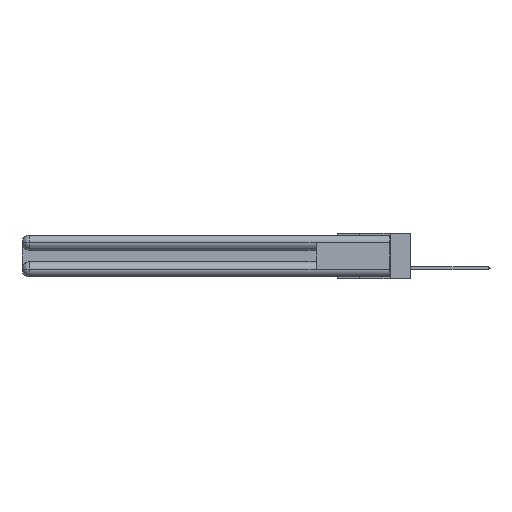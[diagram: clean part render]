
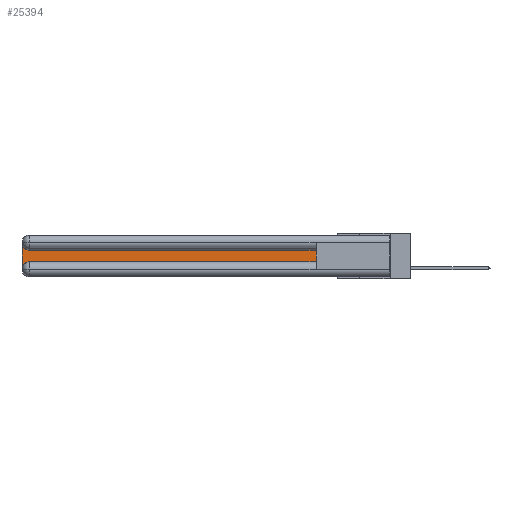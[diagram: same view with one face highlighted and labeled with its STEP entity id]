
A CAD part, left-side view. The second image highlights one B-rep face of the part: STEP entity #25394.
In plain terms, the highlighted planar face has unit normal (-1, 0, 0).
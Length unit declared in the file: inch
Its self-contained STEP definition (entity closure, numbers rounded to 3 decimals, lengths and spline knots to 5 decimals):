
#742 = EDGE_CURVE ( 'NONE', #34128, #25269, #19735, .T. ) ;
#1373 = CARTESIAN_POINT ( 'NONE',  ( 0.075, 0.6, -0.2175 ) ) ;
#2922 = CARTESIAN_POINT ( 'NONE',  ( 0.075, 2.94, -0.2775 ) ) ;
#3399 = EDGE_CURVE ( 'NONE', #27172, #23442, #25266, .T. ) ;
#3717 = CARTESIAN_POINT ( 'NONE',  ( 0.075, 2.94, -0.1225 ) ) ;
#5061 = PLANE ( 'NONE',  #16644 ) ;
#5287 = DIRECTION ( 'NONE',  ( 1., 0., 0. ) ) ;
#5571 = VECTOR ( 'NONE', #8689, 39.37008 ) ;
#6315 = EDGE_CURVE ( 'NONE', #23442, #30089, #26375, .T. ) ;
#6665 = VECTOR ( 'NONE', #15115, 39.37008 ) ;
#6701 = EDGE_LOOP ( 'NONE', ( #14783, #18840, #34577, #16393, #15632, #17587 ) ) ;
#7006 = LINE ( 'NONE', #33624, #23339 ) ;
#8344 = VECTOR ( 'NONE', #23340, 39.37008 ) ;
#8689 = DIRECTION ( 'NONE',  ( 0., 0., 1. ) ) ;
#8804 = CARTESIAN_POINT ( 'NONE',  ( 0.075, 0.6, -0.2175 ) ) ;
#8907 = EDGE_CURVE ( 'NONE', #21850, #34128, #7006, .T. ) ;
#9741 = DIRECTION ( 'NONE',  ( 0., 0., -1. ) ) ;
#9824 = CARTESIAN_POINT ( 'NONE',  ( 0.075, 3., -0.0625 ) ) ;
#10028 = LINE ( 'NONE', #31254, #8344 ) ;
#13073 = EDGE_CURVE ( 'NONE', #25269, #27172, #10028, .T. ) ;
#13792 = DIRECTION ( 'NONE',  ( 1., 0., 0. ) ) ;
#14783 = ORIENTED_EDGE ( 'NONE', *, *, #6315, .T. ) ;
#15115 = DIRECTION ( 'NONE',  ( 0., 1., 0. ) ) ;
#15632 = ORIENTED_EDGE ( 'NONE', *, *, #13073, .T. ) ;
#16393 = ORIENTED_EDGE ( 'NONE', *, *, #742, .T. ) ;
#16644 = AXIS2_PLACEMENT_3D ( 'NONE', #21360, #5287, #23917 ) ;
#17384 = CIRCLE ( 'NONE', #30616, 0.06 ) ;
#17587 = ORIENTED_EDGE ( 'NONE', *, *, #3399, .T. ) ;
#17936 = CARTESIAN_POINT ( 'NONE',  ( 0.075, 0.6, -0.1225 ) ) ;
#18840 = ORIENTED_EDGE ( 'NONE', *, *, #20737, .T. ) ;
#18875 = DIRECTION ( 'NONE',  ( 0., 0., -1. ) ) ;
#19049 = CARTESIAN_POINT ( 'NONE',  ( 0.075, 2.94, -0.2175 ) ) ;
#19735 = CIRCLE ( 'NONE', #23919, 0.06 ) ;
#20353 = DIRECTION ( 'NONE',  ( 0., 0., -1. ) ) ;
#20549 = CARTESIAN_POINT ( 'NONE',  ( 0.075, 2.94, -0.0625 ) ) ;
#20737 = EDGE_CURVE ( 'NONE', #30089, #21850, #17384, .T. ) ;
#21198 = CARTESIAN_POINT ( 'NONE',  ( 0.075, 0.6, -0.1225 ) ) ;
#21360 = CARTESIAN_POINT ( 'NONE',  ( 0.075, 3., -0.1225 ) ) ;
#21850 = VERTEX_POINT ( 'NONE', #9824 ) ;
#23339 = VECTOR ( 'NONE', #20353, 39.37008 ) ;
#23340 = DIRECTION ( 'NONE',  ( 0., -1., 0. ) ) ;
#23442 = VERTEX_POINT ( 'NONE', #21198 ) ;
#23917 = DIRECTION ( 'NONE',  ( 0., 0., -1. ) ) ;
#23919 = AXIS2_PLACEMENT_3D ( 'NONE', #2922, #13792, #18875 ) ;
#25266 = LINE ( 'NONE', #8804, #5571 ) ;
#25269 = VERTEX_POINT ( 'NONE', #19049 ) ;
#25394 = ADVANCED_FACE ( 'NONE', ( #32192 ), #5061, .F. ) ;
#25683 = DIRECTION ( 'NONE',  ( 1., 0., 0. ) ) ;
#26375 = LINE ( 'NONE', #17936, #6665 ) ;
#27172 = VERTEX_POINT ( 'NONE', #1373 ) ;
#29201 = CARTESIAN_POINT ( 'NONE',  ( 0.075, 3., -0.2775 ) ) ;
#30089 = VERTEX_POINT ( 'NONE', #3717 ) ;
#30616 = AXIS2_PLACEMENT_3D ( 'NONE', #20549, #25683, #9741 ) ;
#31254 = CARTESIAN_POINT ( 'NONE',  ( 0.075, 0.6, -0.2175 ) ) ;
#32192 = FACE_OUTER_BOUND ( 'NONE', #6701, .T. ) ;
#33624 = CARTESIAN_POINT ( 'NONE',  ( 0.075, 3., -0.2175 ) ) ;
#34128 = VERTEX_POINT ( 'NONE', #29201 ) ;
#34577 = ORIENTED_EDGE ( 'NONE', *, *, #8907, .T. ) ;
